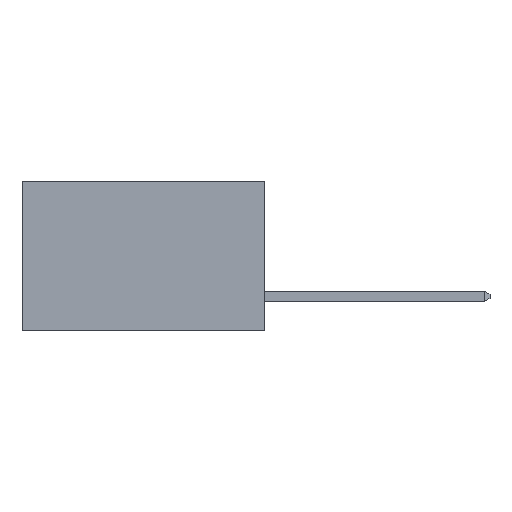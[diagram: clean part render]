
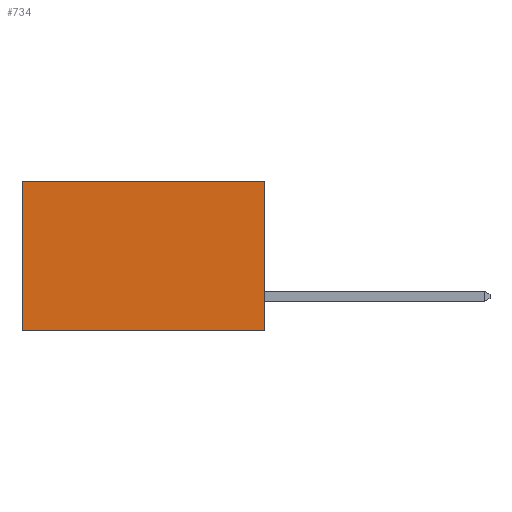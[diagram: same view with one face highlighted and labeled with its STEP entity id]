
A CAD part, left-side view. The second image highlights one B-rep face of the part: STEP entity #734.
In plain terms, the highlighted planar face has unit normal (-1, 0, 0).
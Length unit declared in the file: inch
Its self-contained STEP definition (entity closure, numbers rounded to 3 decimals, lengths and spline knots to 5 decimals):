
#7 = CARTESIAN_POINT ( 'NONE',  ( 0.2615, 0.6, 0. ) ) ;
#150 = EDGE_LOOP ( 'NONE', ( #446, #933, #7441, #7491 ) ) ;
#335 = CARTESIAN_POINT ( 'NONE',  ( 0.2615, 0., -0.37 ) ) ;
#354 = VECTOR ( 'NONE', #4080, 39.37008 ) ;
#446 = ORIENTED_EDGE ( 'NONE', *, *, #3358, .T. ) ;
#734 = ADVANCED_FACE ( 'NONE', ( #1099 ), #8711, .F. ) ;
#849 = VERTEX_POINT ( 'NONE', #9641 ) ;
#933 = ORIENTED_EDGE ( 'NONE', *, *, #8833, .F. ) ;
#1028 = EDGE_CURVE ( 'NONE', #849, #8615, #3497, .T. ) ;
#1071 = VERTEX_POINT ( 'NONE', #4350 ) ;
#1099 = FACE_OUTER_BOUND ( 'NONE', #150, .T. ) ;
#2307 = CARTESIAN_POINT ( 'NONE',  ( 0.2615, 0.6, -0.37 ) ) ;
#2852 = LINE ( 'NONE', #3970, #354 ) ;
#3026 = VERTEX_POINT ( 'NONE', #4341 ) ;
#3358 = EDGE_CURVE ( 'NONE', #8615, #3026, #4403, .T. ) ;
#3497 = LINE ( 'NONE', #9276, #9796 ) ;
#3555 = DIRECTION ( 'NONE',  ( 0., 0., -1. ) ) ;
#3970 = CARTESIAN_POINT ( 'NONE',  ( 0.2615, 0., -0.37 ) ) ;
#4035 = CARTESIAN_POINT ( 'NONE',  ( 0.2615, 0., -0.37 ) ) ;
#4080 = DIRECTION ( 'NONE',  ( 0., 0., -1. ) ) ;
#4341 = CARTESIAN_POINT ( 'NONE',  ( 0.2615, 0.6, -0.37 ) ) ;
#4350 = CARTESIAN_POINT ( 'NONE',  ( 0.2615, 0., -0.37 ) ) ;
#4403 = LINE ( 'NONE', #2307, #8539 ) ;
#4850 = VECTOR ( 'NONE', #8965, 39.37008 ) ;
#4913 = DIRECTION ( 'NONE',  ( 0., 1., 0. ) ) ;
#5018 = EDGE_CURVE ( 'NONE', #849, #1071, #2852, .T. ) ;
#7085 = LINE ( 'NONE', #4035, #4850 ) ;
#7441 = ORIENTED_EDGE ( 'NONE', *, *, #5018, .F. ) ;
#7491 = ORIENTED_EDGE ( 'NONE', *, *, #1028, .T. ) ;
#8393 = DIRECTION ( 'NONE',  ( 1., 0., 0. ) ) ;
#8539 = VECTOR ( 'NONE', #10588, 39.37008 ) ;
#8615 = VERTEX_POINT ( 'NONE', #7 ) ;
#8711 = PLANE ( 'NONE',  #10108 ) ;
#8833 = EDGE_CURVE ( 'NONE', #1071, #3026, #7085, .T. ) ;
#8965 = DIRECTION ( 'NONE',  ( 0., 1., 0. ) ) ;
#9276 = CARTESIAN_POINT ( 'NONE',  ( 0.2615, 0., 0. ) ) ;
#9641 = CARTESIAN_POINT ( 'NONE',  ( 0.2615, 0., 0. ) ) ;
#9796 = VECTOR ( 'NONE', #4913, 39.37008 ) ;
#10108 = AXIS2_PLACEMENT_3D ( 'NONE', #335, #8393, #3555 ) ;
#10588 = DIRECTION ( 'NONE',  ( 0., 0., -1. ) ) ;
